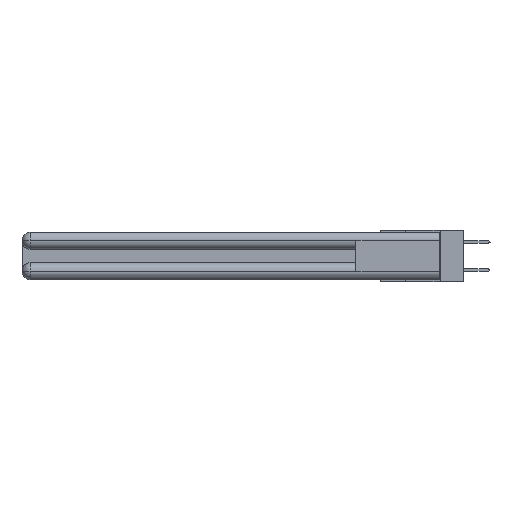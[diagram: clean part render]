
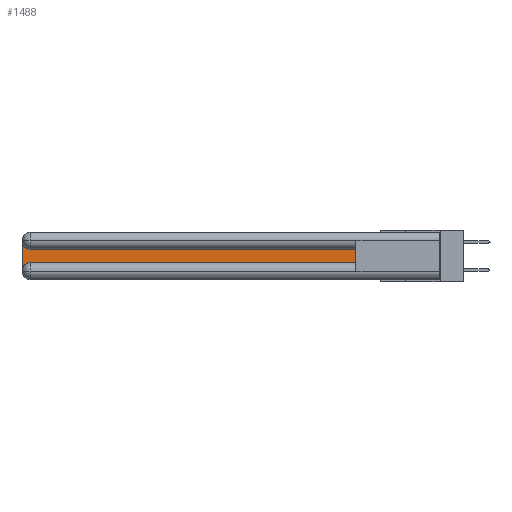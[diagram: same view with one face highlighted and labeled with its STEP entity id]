
A CAD part, left-side view. The second image highlights one B-rep face of the part: STEP entity #1488.
In plain terms, the highlighted planar face has unit normal (-1, 0, 0).
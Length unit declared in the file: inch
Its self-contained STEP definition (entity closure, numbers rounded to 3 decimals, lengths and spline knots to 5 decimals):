
#526 = DIRECTION ( 'NONE',  ( 0., 0., -1. ) ) ;
#1488 = ADVANCED_FACE ( 'NONE', ( #13716 ), #4831, .F. ) ;
#1775 = AXIS2_PLACEMENT_3D ( 'NONE', #25452, #3199, #6253 ) ;
#2424 = CARTESIAN_POINT ( 'NONE',  ( 0.075, 2.94, -0.1225 ) ) ;
#3199 = DIRECTION ( 'NONE',  ( 1., 0., 0. ) ) ;
#3213 = EDGE_CURVE ( 'NONE', #15833, #7770, #9280, .T. ) ;
#3288 = VERTEX_POINT ( 'NONE', #27886 ) ;
#3940 = CARTESIAN_POINT ( 'NONE',  ( 0.075, 3., -0.0625 ) ) ;
#4359 = CARTESIAN_POINT ( 'NONE',  ( 0.075, 0.6, -0.2175 ) ) ;
#4452 = ORIENTED_EDGE ( 'NONE', *, *, #27921, .T. ) ;
#4816 = VECTOR ( 'NONE', #24527, 39.37008 ) ;
#4831 = PLANE ( 'NONE',  #25025 ) ;
#5302 = CARTESIAN_POINT ( 'NONE',  ( 0.075, 0.6, -0.1225 ) ) ;
#6253 = DIRECTION ( 'NONE',  ( 0., 0., -1. ) ) ;
#6480 = ORIENTED_EDGE ( 'NONE', *, *, #7428, .T. ) ;
#7428 = EDGE_CURVE ( 'NONE', #7770, #15113, #17901, .T. ) ;
#7770 = VERTEX_POINT ( 'NONE', #3940 ) ;
#8039 = AXIS2_PLACEMENT_3D ( 'NONE', #13774, #30232, #13647 ) ;
#8499 = LINE ( 'NONE', #22836, #12802 ) ;
#9113 = EDGE_CURVE ( 'NONE', #28222, #13124, #18169, .T. ) ;
#9280 = CIRCLE ( 'NONE', #8039, 0.06 ) ;
#9669 = ORIENTED_EDGE ( 'NONE', *, *, #28394, .T. ) ;
#10920 = CARTESIAN_POINT ( 'NONE',  ( 0.075, 0.6, -0.2175 ) ) ;
#11595 = CARTESIAN_POINT ( 'NONE',  ( 0.075, 3., -0.1225 ) ) ;
#12802 = VECTOR ( 'NONE', #17144, 39.37008 ) ;
#13124 = VERTEX_POINT ( 'NONE', #10920 ) ;
#13540 = CARTESIAN_POINT ( 'NONE',  ( 0.075, 3., -0.2175 ) ) ;
#13647 = DIRECTION ( 'NONE',  ( 0., 0., -1. ) ) ;
#13716 = FACE_OUTER_BOUND ( 'NONE', #30573, .T. ) ;
#13774 = CARTESIAN_POINT ( 'NONE',  ( 0.075, 2.94, -0.0625 ) ) ;
#15113 = VERTEX_POINT ( 'NONE', #31984 ) ;
#15157 = VECTOR ( 'NONE', #23970, 39.37008 ) ;
#15833 = VERTEX_POINT ( 'NONE', #2424 ) ;
#16059 = ORIENTED_EDGE ( 'NONE', *, *, #9113, .T. ) ;
#17144 = DIRECTION ( 'NONE',  ( 0., 0., 1. ) ) ;
#17554 = VECTOR ( 'NONE', #18933, 39.37008 ) ;
#17901 = LINE ( 'NONE', #13540, #4816 ) ;
#18169 = LINE ( 'NONE', #4359, #15157 ) ;
#18933 = DIRECTION ( 'NONE',  ( 0., 1., 0. ) ) ;
#19158 = EDGE_CURVE ( 'NONE', #15113, #28222, #19889, .T. ) ;
#19889 = CIRCLE ( 'NONE', #1775, 0.06 ) ;
#20232 = ORIENTED_EDGE ( 'NONE', *, *, #3213, .T. ) ;
#22335 = ORIENTED_EDGE ( 'NONE', *, *, #19158, .T. ) ;
#22836 = CARTESIAN_POINT ( 'NONE',  ( 0.075, 0.6, -0.2175 ) ) ;
#23970 = DIRECTION ( 'NONE',  ( 0., -1., 0. ) ) ;
#24527 = DIRECTION ( 'NONE',  ( 0., 0., -1. ) ) ;
#25025 = AXIS2_PLACEMENT_3D ( 'NONE', #11595, #31468, #526 ) ;
#25452 = CARTESIAN_POINT ( 'NONE',  ( 0.075, 2.94, -0.2775 ) ) ;
#27886 = CARTESIAN_POINT ( 'NONE',  ( 0.075, 0.6, -0.1225 ) ) ;
#27921 = EDGE_CURVE ( 'NONE', #13124, #3288, #8499, .T. ) ;
#28222 = VERTEX_POINT ( 'NONE', #32251 ) ;
#28394 = EDGE_CURVE ( 'NONE', #3288, #15833, #33293, .T. ) ;
#30232 = DIRECTION ( 'NONE',  ( 1., 0., 0. ) ) ;
#30573 = EDGE_LOOP ( 'NONE', ( #9669, #20232, #6480, #22335, #16059, #4452 ) ) ;
#31468 = DIRECTION ( 'NONE',  ( 1., 0., 0. ) ) ;
#31984 = CARTESIAN_POINT ( 'NONE',  ( 0.075, 3., -0.2775 ) ) ;
#32251 = CARTESIAN_POINT ( 'NONE',  ( 0.075, 2.94, -0.2175 ) ) ;
#33293 = LINE ( 'NONE', #5302, #17554 ) ;
